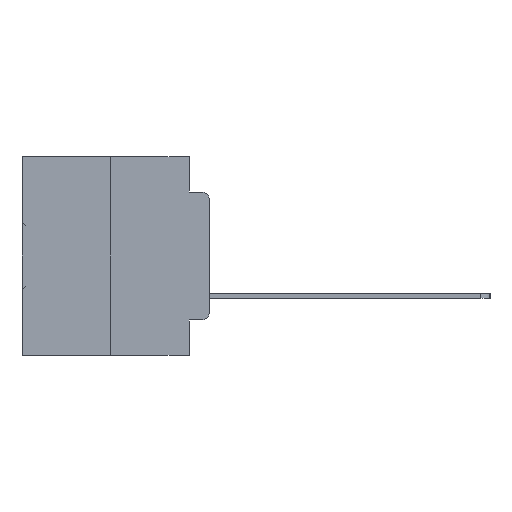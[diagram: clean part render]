
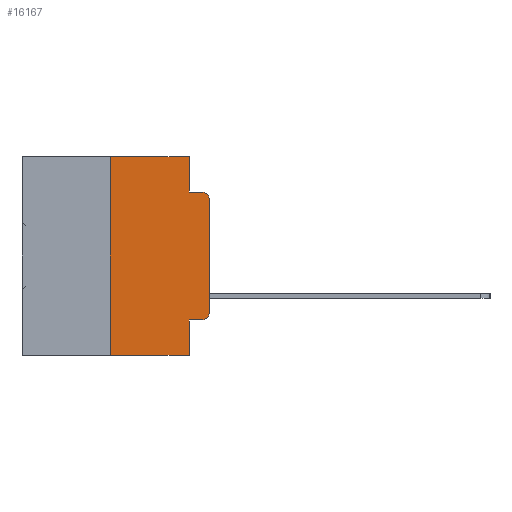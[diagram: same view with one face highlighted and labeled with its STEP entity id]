
A CAD part, left-side view. The second image highlights one B-rep face of the part: STEP entity #16167.
In plain terms, the highlighted planar face has unit normal (-1, 0, 0).
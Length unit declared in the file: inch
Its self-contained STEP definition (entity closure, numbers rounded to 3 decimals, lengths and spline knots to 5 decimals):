
#32 = CARTESIAN_POINT ( 'NONE',  ( 0., 0., 0. ) ) ;
#579 = VECTOR ( 'NONE', #15576, 39.37008 ) ;
#770 = CARTESIAN_POINT ( 'NONE',  ( 0., 0.051, 0. ) ) ;
#1237 = CARTESIAN_POINT ( 'NONE',  ( 0., 0.25, 0. ) ) ;
#2018 = ORIENTED_EDGE ( 'NONE', *, *, #23129, .T. ) ;
#2571 = CARTESIAN_POINT ( 'NONE',  ( 0., 0.473, 0. ) ) ;
#3269 = VECTOR ( 'NONE', #7716, 39.37008 ) ;
#3305 = CARTESIAN_POINT ( 'NONE',  ( 0., 0.051, 0. ) ) ;
#3406 = CARTESIAN_POINT ( 'NONE',  ( 0., 0., -0.1085 ) ) ;
#3978 = DIRECTION ( 'NONE',  ( -1., 0., 0. ) ) ;
#6161 = DIRECTION ( 'NONE',  ( 0., 0., -1. ) ) ;
#6414 = EDGE_LOOP ( 'NONE', ( #6880, #2018, #19663, #17211, #8984, #12473, #15239, #15002, #14079, #21365 ) ) ;
#6598 = LINE ( 'NONE', #1237, #13925 ) ;
#6606 = EDGE_CURVE ( 'NONE', #8214, #18597, #18066, .T. ) ;
#6880 = ORIENTED_EDGE ( 'NONE', *, *, #24940, .T. ) ;
#7261 = VECTOR ( 'NONE', #20361, 39.37008 ) ;
#7268 = PLANE ( 'NONE',  #11529 ) ;
#7716 = DIRECTION ( 'NONE',  ( 0., -1., 0. ) ) ;
#7992 = AXIS2_PLACEMENT_3D ( 'NONE', #30535, #14310, #33208 ) ;
#8214 = VERTEX_POINT ( 'NONE', #10841 ) ;
#8515 = EDGE_CURVE ( 'NONE', #27345, #8214, #20953, .T. ) ;
#8984 = ORIENTED_EDGE ( 'NONE', *, *, #12441, .F. ) ;
#9533 = VERTEX_POINT ( 'NONE', #13449 ) ;
#10058 = DIRECTION ( 'NONE',  ( 1., 0., 0. ) ) ;
#10346 = EDGE_CURVE ( 'NONE', #27345, #31304, #26799, .T. ) ;
#10841 = CARTESIAN_POINT ( 'NONE',  ( 0., 0.02, -0.4115 ) ) ;
#10847 = VECTOR ( 'NONE', #27670, 39.37008 ) ;
#11405 = CARTESIAN_POINT ( 'NONE',  ( 0., 0.051, 0. ) ) ;
#11501 = VERTEX_POINT ( 'NONE', #27931 ) ;
#11529 = AXIS2_PLACEMENT_3D ( 'NONE', #18175, #10058, #29086 ) ;
#12441 = EDGE_CURVE ( 'NONE', #27792, #23210, #35416, .T. ) ;
#12473 = ORIENTED_EDGE ( 'NONE', *, *, #13988, .F. ) ;
#13449 = CARTESIAN_POINT ( 'NONE',  ( 0., 0.051, -0.0885 ) ) ;
#13925 = VECTOR ( 'NONE', #20570, 39.37008 ) ;
#13988 = EDGE_CURVE ( 'NONE', #11501, #27792, #6598, .T. ) ;
#14079 = ORIENTED_EDGE ( 'NONE', *, *, #8515, .T. ) ;
#14271 = CIRCLE ( 'NONE', #7992, 0.02 ) ;
#14310 = DIRECTION ( 'NONE',  ( -1., 0., 0. ) ) ;
#15001 = CARTESIAN_POINT ( 'NONE',  ( 0., 0.051, -0.4115 ) ) ;
#15002 = ORIENTED_EDGE ( 'NONE', *, *, #10346, .F. ) ;
#15239 = ORIENTED_EDGE ( 'NONE', *, *, #18129, .T. ) ;
#15391 = CARTESIAN_POINT ( 'NONE',  ( 0., 0.051, -0.4115 ) ) ;
#15576 = DIRECTION ( 'NONE',  ( 0., -1., 0. ) ) ;
#15824 = EDGE_CURVE ( 'NONE', #23210, #9533, #32461, .T. ) ;
#16167 = ADVANCED_FACE ( 'NONE', ( #28699 ), #7268, .F. ) ;
#17211 = ORIENTED_EDGE ( 'NONE', *, *, #15824, .F. ) ;
#17678 = EDGE_CURVE ( 'NONE', #9533, #18970, #34823, .T. ) ;
#18066 = CIRCLE ( 'NONE', #24278, 0.02 ) ;
#18129 = EDGE_CURVE ( 'NONE', #11501, #31304, #29792, .T. ) ;
#18175 = CARTESIAN_POINT ( 'NONE',  ( 0., 0.473, 0. ) ) ;
#18597 = VERTEX_POINT ( 'NONE', #28367 ) ;
#18970 = VERTEX_POINT ( 'NONE', #27272 ) ;
#19311 = VECTOR ( 'NONE', #19426, 39.37008 ) ;
#19426 = DIRECTION ( 'NONE',  ( 0., 0., 1. ) ) ;
#19663 = ORIENTED_EDGE ( 'NONE', *, *, #17678, .F. ) ;
#20361 = DIRECTION ( 'NONE',  ( 0., -1., 0. ) ) ;
#20450 = VECTOR ( 'NONE', #6161, 39.37008 ) ;
#20483 = CARTESIAN_POINT ( 'NONE',  ( 0., 0.02, -0.3915 ) ) ;
#20570 = DIRECTION ( 'NONE',  ( 0., 0., 1. ) ) ;
#20953 = LINE ( 'NONE', #15001, #7261 ) ;
#21305 = CARTESIAN_POINT ( 'NONE',  ( 0., 0.051, -0.0885 ) ) ;
#21365 = ORIENTED_EDGE ( 'NONE', *, *, #6606, .T. ) ;
#21852 = DIRECTION ( 'NONE',  ( 0., -1., 0. ) ) ;
#21981 = VECTOR ( 'NONE', #21852, 39.37008 ) ;
#23129 = EDGE_CURVE ( 'NONE', #24479, #18970, #14271, .T. ) ;
#23210 = VERTEX_POINT ( 'NONE', #770 ) ;
#23221 = DIRECTION ( 'NONE',  ( 0., 0., -1. ) ) ;
#24278 = AXIS2_PLACEMENT_3D ( 'NONE', #20483, #3978, #23221 ) ;
#24479 = VERTEX_POINT ( 'NONE', #3406 ) ;
#24816 = LINE ( 'NONE', #32, #19311 ) ;
#24940 = EDGE_CURVE ( 'NONE', #18597, #24479, #24816, .T. ) ;
#25012 = CARTESIAN_POINT ( 'NONE',  ( 0., 0.051, -0.5 ) ) ;
#26799 = LINE ( 'NONE', #3305, #20450 ) ;
#27272 = CARTESIAN_POINT ( 'NONE',  ( 0., 0.02, -0.0885 ) ) ;
#27345 = VERTEX_POINT ( 'NONE', #15391 ) ;
#27670 = DIRECTION ( 'NONE',  ( 0., 0., -1. ) ) ;
#27792 = VERTEX_POINT ( 'NONE', #28409 ) ;
#27931 = CARTESIAN_POINT ( 'NONE',  ( 0., 0.25, -0.5 ) ) ;
#28367 = CARTESIAN_POINT ( 'NONE',  ( 0., 0., -0.3915 ) ) ;
#28409 = CARTESIAN_POINT ( 'NONE',  ( 0., 0.25, 0. ) ) ;
#28699 = FACE_OUTER_BOUND ( 'NONE', #6414, .T. ) ;
#29086 = DIRECTION ( 'NONE',  ( 0., 0., -1. ) ) ;
#29121 = CARTESIAN_POINT ( 'NONE',  ( 0., 0.473, -0.5 ) ) ;
#29792 = LINE ( 'NONE', #29121, #579 ) ;
#30535 = CARTESIAN_POINT ( 'NONE',  ( 0., 0.02, -0.1085 ) ) ;
#31304 = VERTEX_POINT ( 'NONE', #25012 ) ;
#32461 = LINE ( 'NONE', #11405, #10847 ) ;
#33208 = DIRECTION ( 'NONE',  ( 0., 0., -1. ) ) ;
#34823 = LINE ( 'NONE', #21305, #3269 ) ;
#35416 = LINE ( 'NONE', #2571, #21981 ) ;
